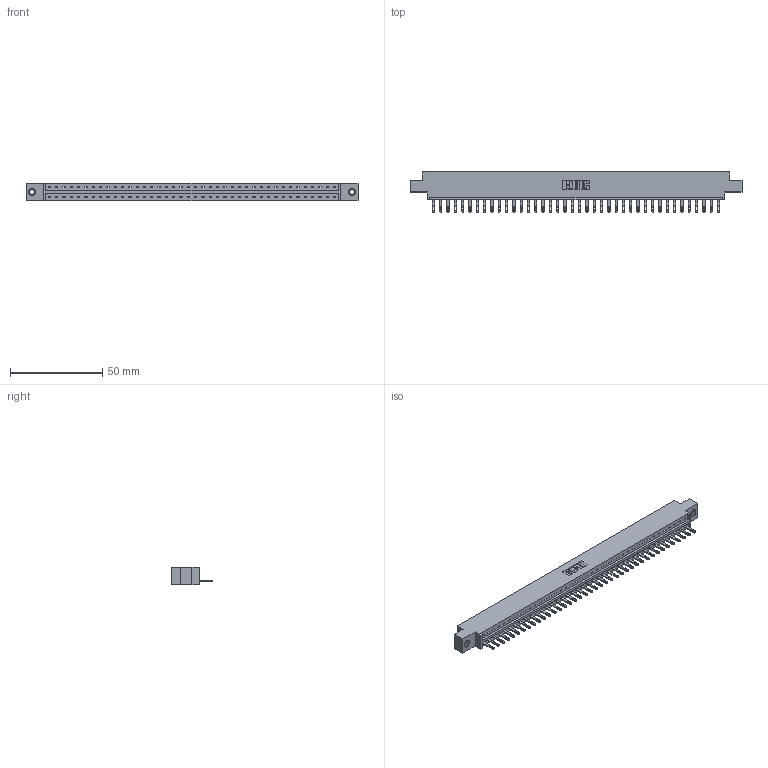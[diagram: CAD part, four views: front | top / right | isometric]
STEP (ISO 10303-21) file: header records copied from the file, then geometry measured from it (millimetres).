
FILE_DESCRIPTION (( 'STEP AP203' ), '1' );
FILE_NAME ('333-040-500-607.STEP', '2018-08-03T13:25:16', ( '' ), ( '' ), 'SwSTEP 2.0', 'SolidWorks 2016', '' );
FILE_SCHEMA (( 'CONFIG_CONTROL_DESIGN' ));
Length unit declared in the file: inch
Products named in the file (4): 333 Part_Offset - .156 Dia - TI; 345-292-001_345-293-100; 345-250-001_345-250-005-103; 333-040-500-607
Assembly tree (43 placements, depth 2):
  333-040-500-607
    333 Part_Offset - .156 Dia - TI
    345-292-001_345-293-100  x40
    345-250-001_345-250-005-103  x2
Bounding box: 180.04 x 21.85 x 9.4 mm (x, y, z)
Volume: 17882.9 mm3; surface area: 19668.6 mm2
Topology: 43 solids, 43 shells, 2338 faces, 7179 edges, 4778 vertices
Faces by surface type: plane 1546, cylinder 776, cone 12, torus 4
Entity records: 25960 total; most frequent: CARTESIAN_POINT 4461, ORIENTED_EDGE 4430, DIRECTION 3801, EDGE_CURVE 2215, VECTOR 2063, LINE 2063, VERTEX_POINT 1472, AXIS2_PLACEMENT_3D 869
